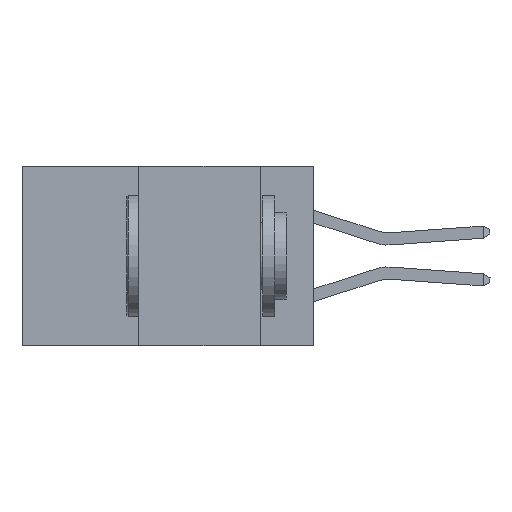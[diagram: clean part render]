
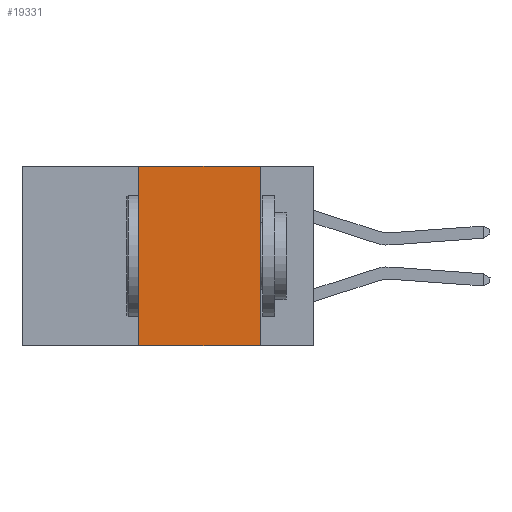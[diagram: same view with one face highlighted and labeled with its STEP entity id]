
A CAD part, left-side view. The second image highlights one B-rep face of the part: STEP entity #19331.
In plain terms, the highlighted planar face has unit normal (-1, 0, 0).
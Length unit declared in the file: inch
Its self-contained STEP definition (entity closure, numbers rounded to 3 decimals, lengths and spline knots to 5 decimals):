
#637 = CARTESIAN_POINT ( 'NONE',  ( 0., 0.36, 0. ) ) ;
#1302 = DIRECTION ( 'NONE',  ( 0., -1., 0. ) ) ;
#2210 = CARTESIAN_POINT ( 'NONE',  ( 0., 0.11, 0. ) ) ;
#2317 = ORIENTED_EDGE ( 'NONE', *, *, #16507, .F. ) ;
#2468 = DIRECTION ( 'NONE',  ( 0., 0., -1. ) ) ;
#2860 = CARTESIAN_POINT ( 'NONE',  ( 0., 0.11, -0.37 ) ) ;
#3121 = ORIENTED_EDGE ( 'NONE', *, *, #19671, .F. ) ;
#4131 = AXIS2_PLACEMENT_3D ( 'NONE', #16577, #23245, #2468 ) ;
#4711 = ORIENTED_EDGE ( 'NONE', *, *, #19854, .T. ) ;
#5527 = CARTESIAN_POINT ( 'NONE',  ( 0., 0.6, 0. ) ) ;
#5568 = VERTEX_POINT ( 'NONE', #8950 ) ;
#7082 = VECTOR ( 'NONE', #25445, 39.37008 ) ;
#7291 = VECTOR ( 'NONE', #25572, 39.37008 ) ;
#7666 = LINE ( 'NONE', #28072, #7291 ) ;
#8049 = FACE_OUTER_BOUND ( 'NONE', #15753, .T. ) ;
#8950 = CARTESIAN_POINT ( 'NONE',  ( 0., 0.36, -0.37 ) ) ;
#13168 = VECTOR ( 'NONE', #1302, 39.37008 ) ;
#13191 = VERTEX_POINT ( 'NONE', #26151 ) ;
#14578 = LINE ( 'NONE', #5527, #13168 ) ;
#15048 = LINE ( 'NONE', #2210, #7082 ) ;
#15399 = DIRECTION ( 'NONE',  ( 0., 0., 1. ) ) ;
#15753 = EDGE_LOOP ( 'NONE', ( #26408, #3121, #2317, #4711 ) ) ;
#16228 = LINE ( 'NONE', #24520, #21617 ) ;
#16507 = EDGE_CURVE ( 'NONE', #5568, #18878, #16228, .T. ) ;
#16577 = CARTESIAN_POINT ( 'NONE',  ( 0., 0.6, 0. ) ) ;
#18878 = VERTEX_POINT ( 'NONE', #637 ) ;
#19331 = ADVANCED_FACE ( 'NONE', ( #8049 ), #27502, .F. ) ;
#19671 = EDGE_CURVE ( 'NONE', #18878, #13191, #14578, .T. ) ;
#19854 = EDGE_CURVE ( 'NONE', #5568, #25160, #7666, .T. ) ;
#21617 = VECTOR ( 'NONE', #15399, 39.37008 ) ;
#22488 = EDGE_CURVE ( 'NONE', #13191, #25160, #15048, .T. ) ;
#23245 = DIRECTION ( 'NONE',  ( 1., 0., 0. ) ) ;
#24520 = CARTESIAN_POINT ( 'NONE',  ( 0., 0.36, 0. ) ) ;
#25160 = VERTEX_POINT ( 'NONE', #2860 ) ;
#25445 = DIRECTION ( 'NONE',  ( 0., 0., -1. ) ) ;
#25572 = DIRECTION ( 'NONE',  ( 0., -1., 0. ) ) ;
#26151 = CARTESIAN_POINT ( 'NONE',  ( 0., 0.11, 0. ) ) ;
#26408 = ORIENTED_EDGE ( 'NONE', *, *, #22488, .F. ) ;
#27502 = PLANE ( 'NONE',  #4131 ) ;
#28072 = CARTESIAN_POINT ( 'NONE',  ( 0., 0.6, -0.37 ) ) ;
